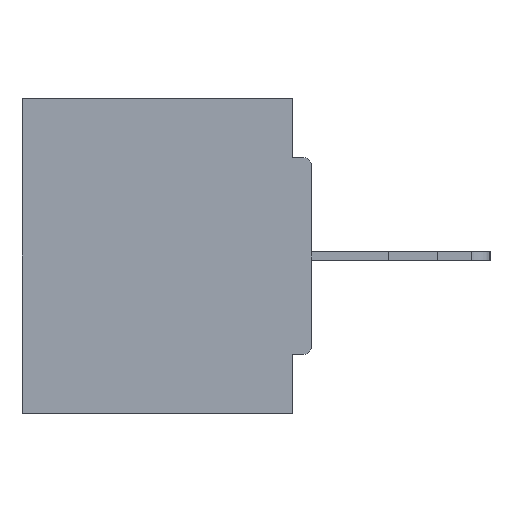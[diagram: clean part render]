
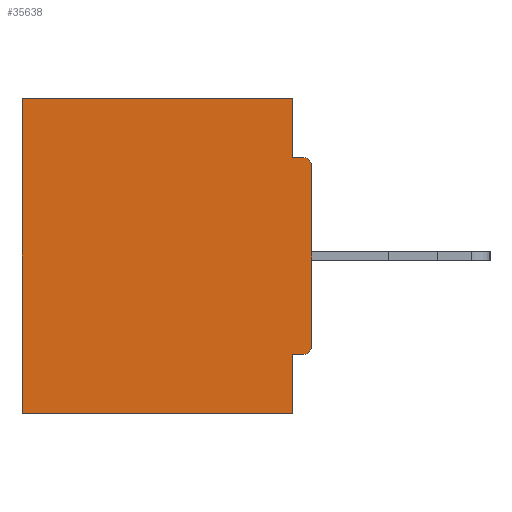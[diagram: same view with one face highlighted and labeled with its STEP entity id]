
A CAD part, left-side view. The second image highlights one B-rep face of the part: STEP entity #35638.
In plain terms, the highlighted planar face has unit normal (-1, 0, 0).
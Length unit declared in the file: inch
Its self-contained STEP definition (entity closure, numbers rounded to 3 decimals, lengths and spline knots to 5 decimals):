
#752 = CARTESIAN_POINT ( 'NONE',  ( 0.298, 0.46, 0. ) ) ;
#917 = EDGE_CURVE ( 'NONE', #31319, #9860, #17304, .T. ) ;
#1192 = DIRECTION ( 'NONE',  ( 0., 0., -1. ) ) ;
#1235 = CARTESIAN_POINT ( 'NONE',  ( 0.298, 0.015, -0.1085 ) ) ;
#1238 = DIRECTION ( 'NONE',  ( -1., 0., 0. ) ) ;
#1485 = LINE ( 'NONE', #8066, #11140 ) ;
#1953 = AXIS2_PLACEMENT_3D ( 'NONE', #1235, #1238, #1192 ) ;
#2256 = PLANE ( 'NONE',  #8738 ) ;
#2524 = VERTEX_POINT ( 'NONE', #9077 ) ;
#2527 = DIRECTION ( 'NONE',  ( 0., 0., -1. ) ) ;
#2628 = LINE ( 'NONE', #26044, #24822 ) ;
#3127 = ORIENTED_EDGE ( 'NONE', *, *, #17229, .T. ) ;
#3277 = CARTESIAN_POINT ( 'NONE',  ( 0.298, 0.031, -0.5 ) ) ;
#3537 = CARTESIAN_POINT ( 'NONE',  ( 0.298, 0., -0.3915 ) ) ;
#3632 = LINE ( 'NONE', #12038, #25747 ) ;
#3828 = ORIENTED_EDGE ( 'NONE', *, *, #19091, .F. ) ;
#4739 = EDGE_CURVE ( 'NONE', #8805, #30453, #24660, .T. ) ;
#6982 = ORIENTED_EDGE ( 'NONE', *, *, #29488, .F. ) ;
#7589 = VERTEX_POINT ( 'NONE', #26381 ) ;
#7829 = EDGE_CURVE ( 'NONE', #31319, #32223, #21760, .T. ) ;
#7858 = CIRCLE ( 'NONE', #8804, 0.015 ) ;
#8066 = CARTESIAN_POINT ( 'NONE',  ( 0.298, 0., -0.0935 ) ) ;
#8230 = LINE ( 'NONE', #20763, #20776 ) ;
#8236 = DIRECTION ( 'NONE',  ( 1., 0., 0. ) ) ;
#8570 = ORIENTED_EDGE ( 'NONE', *, *, #4739, .T. ) ;
#8690 = ORIENTED_EDGE ( 'NONE', *, *, #7829, .F. ) ;
#8738 = AXIS2_PLACEMENT_3D ( 'NONE', #16771, #8236, #28286 ) ;
#8804 = AXIS2_PLACEMENT_3D ( 'NONE', #37082, #19900, #2527 ) ;
#8805 = VERTEX_POINT ( 'NONE', #10645 ) ;
#9077 = CARTESIAN_POINT ( 'NONE',  ( 0.298, 0.031, -0.0935 ) ) ;
#9193 = DIRECTION ( 'NONE',  ( 0., 0., -1. ) ) ;
#9860 = VERTEX_POINT ( 'NONE', #26726 ) ;
#10645 = CARTESIAN_POINT ( 'NONE',  ( 0.298, 0.031, 0. ) ) ;
#11140 = VECTOR ( 'NONE', #33926, 39.37008 ) ;
#11330 = EDGE_CURVE ( 'NONE', #8805, #2524, #8230, .T. ) ;
#11576 = CARTESIAN_POINT ( 'NONE',  ( 0.298, 0., 0. ) ) ;
#11806 = LINE ( 'NONE', #21257, #33807 ) ;
#12038 = CARTESIAN_POINT ( 'NONE',  ( 0.298, 0., -0.4065 ) ) ;
#12920 = ORIENTED_EDGE ( 'NONE', *, *, #18660, .F. ) ;
#13316 = ORIENTED_EDGE ( 'NONE', *, *, #15871, .F. ) ;
#15871 = EDGE_CURVE ( 'NONE', #36038, #19830, #33932, .T. ) ;
#16435 = CARTESIAN_POINT ( 'NONE',  ( 0.298, 0.015, -0.4065 ) ) ;
#16771 = CARTESIAN_POINT ( 'NONE',  ( 0.298, 0., 0. ) ) ;
#16912 = ORIENTED_EDGE ( 'NONE', *, *, #917, .T. ) ;
#17035 = VECTOR ( 'NONE', #35364, 39.37008 ) ;
#17229 = EDGE_CURVE ( 'NONE', #21558, #32223, #7858, .T. ) ;
#17304 = CIRCLE ( 'NONE', #1953, 0.015 ) ;
#17826 = ORIENTED_EDGE ( 'NONE', *, *, #11330, .F. ) ;
#18660 = EDGE_CURVE ( 'NONE', #21558, #36038, #3632, .T. ) ;
#19091 = EDGE_CURVE ( 'NONE', #19830, #7589, #2628, .T. ) ;
#19248 = EDGE_CURVE ( 'NONE', #30453, #7589, #11806, .T. ) ;
#19830 = VERTEX_POINT ( 'NONE', #20586 ) ;
#19900 = DIRECTION ( 'NONE',  ( -1., 0., 0. ) ) ;
#19908 = CARTESIAN_POINT ( 'NONE',  ( 0.298, 0., -0.1085 ) ) ;
#20391 = DIRECTION ( 'NONE',  ( 0., 1., 0. ) ) ;
#20586 = CARTESIAN_POINT ( 'NONE',  ( 0.298, 0.031, -0.5 ) ) ;
#20763 = CARTESIAN_POINT ( 'NONE',  ( 0.298, 0.031, -0.5 ) ) ;
#20776 = VECTOR ( 'NONE', #23654, 39.37008 ) ;
#21257 = CARTESIAN_POINT ( 'NONE',  ( 0.298, 0.46, 0. ) ) ;
#21558 = VERTEX_POINT ( 'NONE', #16435 ) ;
#21760 = LINE ( 'NONE', #11576, #27596 ) ;
#22522 = DIRECTION ( 'NONE',  ( 0., 0., -1. ) ) ;
#23556 = DIRECTION ( 'NONE',  ( 0., 1., 0. ) ) ;
#23654 = DIRECTION ( 'NONE',  ( 0., 0., -1. ) ) ;
#23897 = EDGE_LOOP ( 'NONE', ( #16912, #6982, #17826, #8570, #28564, #3828, #13316, #12920, #3127, #8690 ) ) ;
#24131 = DIRECTION ( 'NONE',  ( 0., 0., -1. ) ) ;
#24632 = CARTESIAN_POINT ( 'NONE',  ( 0.298, 0.031, -0.4065 ) ) ;
#24660 = LINE ( 'NONE', #33871, #17035 ) ;
#24822 = VECTOR ( 'NONE', #20391, 39.37008 ) ;
#24845 = FACE_OUTER_BOUND ( 'NONE', #23897, .T. ) ;
#25368 = VECTOR ( 'NONE', #9193, 39.37008 ) ;
#25747 = VECTOR ( 'NONE', #23556, 39.37008 ) ;
#26044 = CARTESIAN_POINT ( 'NONE',  ( 0.298, 0., -0.5 ) ) ;
#26381 = CARTESIAN_POINT ( 'NONE',  ( 0.298, 0.46, -0.5 ) ) ;
#26726 = CARTESIAN_POINT ( 'NONE',  ( 0.298, 0.015, -0.0935 ) ) ;
#27596 = VECTOR ( 'NONE', #22522, 39.37008 ) ;
#28286 = DIRECTION ( 'NONE',  ( 0., 0., -1. ) ) ;
#28564 = ORIENTED_EDGE ( 'NONE', *, *, #19248, .T. ) ;
#29488 = EDGE_CURVE ( 'NONE', #2524, #9860, #1485, .T. ) ;
#30453 = VERTEX_POINT ( 'NONE', #752 ) ;
#31319 = VERTEX_POINT ( 'NONE', #19908 ) ;
#32223 = VERTEX_POINT ( 'NONE', #3537 ) ;
#33807 = VECTOR ( 'NONE', #24131, 39.37008 ) ;
#33871 = CARTESIAN_POINT ( 'NONE',  ( 0.298, 0., 0. ) ) ;
#33926 = DIRECTION ( 'NONE',  ( 0., -1., 0. ) ) ;
#33932 = LINE ( 'NONE', #3277, #25368 ) ;
#35364 = DIRECTION ( 'NONE',  ( 0., 1., 0. ) ) ;
#35638 = ADVANCED_FACE ( 'NONE', ( #24845 ), #2256, .F. ) ;
#36038 = VERTEX_POINT ( 'NONE', #24632 ) ;
#37082 = CARTESIAN_POINT ( 'NONE',  ( 0.298, 0.015, -0.3915 ) ) ;
